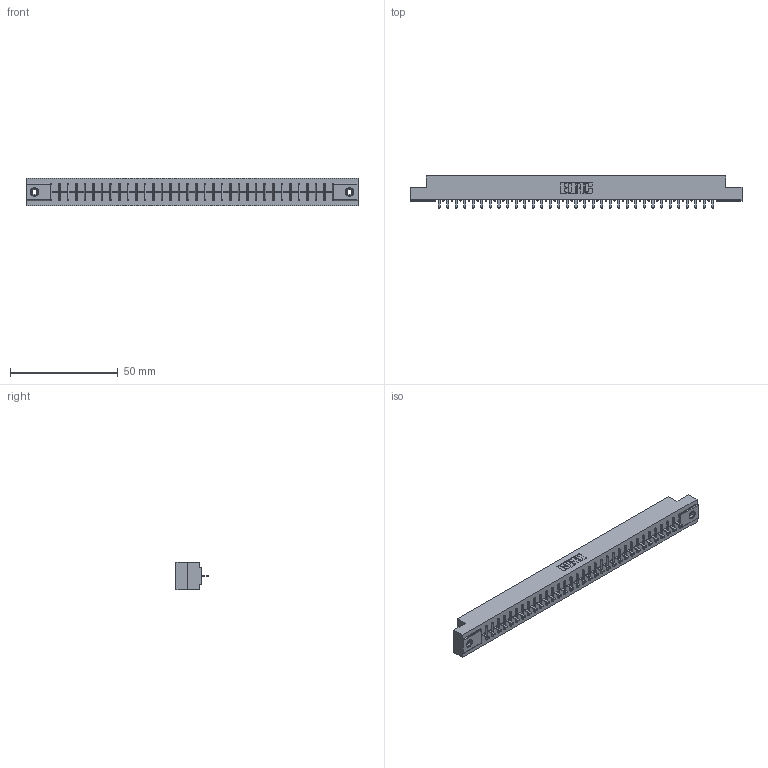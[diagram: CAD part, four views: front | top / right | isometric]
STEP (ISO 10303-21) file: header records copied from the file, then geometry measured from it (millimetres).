
FILE_DESCRIPTION (( 'STEP AP203' ), '1' );
FILE_NAME ('356-033-421-108.STEP', '2020-09-23T21:47:04', ( '' ), ( '' ), 'SwSTEP 2.0', 'SolidWorks 2020', '' );
FILE_SCHEMA (( 'CONFIG_CONTROL_DESIGN' ));
Length unit declared in the file: inch
Products named in the file (4): 306-290-001_121; 306 Part_.156 Dia; 356-033-421-108; 345-250-001_345-250-003-102
Assembly tree (36 placements, depth 2):
  356-033-421-108
    306 Part_.156 Dia
    306-290-001_121  x33
    345-250-001_345-250-003-102  x2
Bounding box: 153.77 x 14.88 x 12.7 mm (x, y, z)
Volume: 16872.2 mm3; surface area: 17007.2 mm2
Topology: 36 solids, 36 shells, 2486 faces, 6953 edges, 4450 vertices
Faces by surface type: plane 1651, cylinder 687, sphere 132, cone 12, torus 4
Entity records: 33081 total; most frequent: CARTESIAN_POINT 5533, ORIENTED_EDGE 5478, DIRECTION 5465, EDGE_CURVE 2739, LINE 2137, VECTOR 2137, VERTEX_POINT 1732, AXIS2_PLACEMENT_3D 1664
